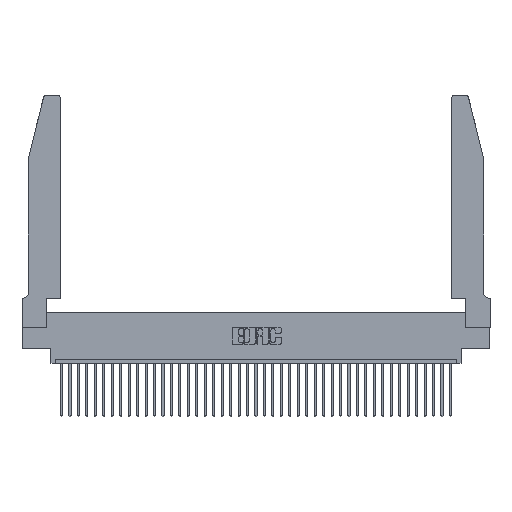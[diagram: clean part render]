
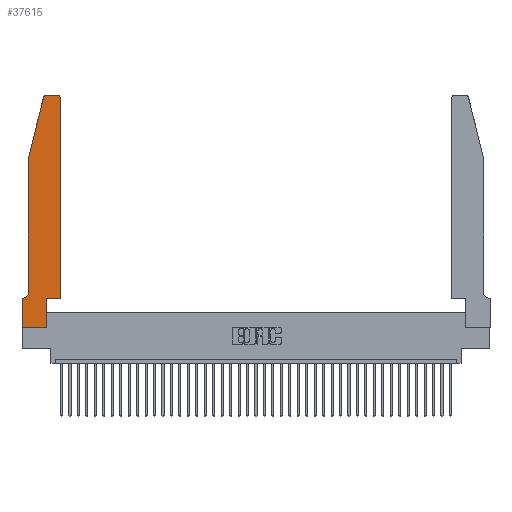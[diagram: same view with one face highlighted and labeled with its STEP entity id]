
A CAD part, top view. The second image highlights one B-rep face of the part: STEP entity #37615.
In plain terms, the highlighted planar face has unit normal (0, 0, 1).
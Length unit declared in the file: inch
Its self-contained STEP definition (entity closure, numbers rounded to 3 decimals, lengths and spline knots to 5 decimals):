
#205 = DIRECTION ( 'NONE',  ( -1., 0., 0. ) ) ;
#298 = EDGE_CURVE ( 'NONE', #4939, #35793, #22184, .T. ) ;
#936 = CARTESIAN_POINT ( 'NONE',  ( 0.0755, 2., 0.37 ) ) ;
#2303 = CARTESIAN_POINT ( 'NONE',  ( 0.284, 2.72, 0.37 ) ) ;
#2521 = CARTESIAN_POINT ( 'NONE',  ( 0.284, 2.75, 0.37 ) ) ;
#3722 = CARTESIAN_POINT ( 'NONE',  ( 0.2865, 0.35, 0.37 ) ) ;
#4431 = VERTEX_POINT ( 'NONE', #35294 ) ;
#4633 = CIRCLE ( 'NONE', #36306, 0.07 ) ;
#4719 = EDGE_CURVE ( 'NONE', #36142, #27491, #20050, .T. ) ;
#4939 = VERTEX_POINT ( 'NONE', #25832 ) ;
#5472 = VECTOR ( 'NONE', #21327, 39.37008 ) ;
#5750 = EDGE_CURVE ( 'NONE', #32243, #20585, #34738, .T. ) ;
#6761 = DIRECTION ( 'NONE',  ( 0., 1., 0. ) ) ;
#7366 = DIRECTION ( 'NONE',  ( -1., 0., 0. ) ) ;
#7475 = PLANE ( 'NONE',  #34757 ) ;
#7503 = DIRECTION ( 'NONE',  ( 1., 0., 0. ) ) ;
#7834 = VECTOR ( 'NONE', #29791, 39.37008 ) ;
#8847 = ORIENTED_EDGE ( 'NONE', *, *, #26041, .T. ) ;
#10154 = CARTESIAN_POINT ( 'NONE',  ( 0.4505, 0.35, 0.37 ) ) ;
#11178 = EDGE_CURVE ( 'NONE', #20585, #12374, #34008, .T. ) ;
#11465 = CARTESIAN_POINT ( 'NONE',  ( 0.0755, 0.35, 0.37 ) ) ;
#11670 = CARTESIAN_POINT ( 'NONE',  ( 0.4505, 0.35, 0.37 ) ) ;
#12374 = VERTEX_POINT ( 'NONE', #31722 ) ;
#12647 = DIRECTION ( 'NONE',  ( 0., -1., 0. ) ) ;
#13326 = EDGE_CURVE ( 'NONE', #36892, #4939, #19471, .T. ) ;
#13401 = VERTEX_POINT ( 'NONE', #14590 ) ;
#13885 = CARTESIAN_POINT ( 'NONE',  ( 0.4205, 2.72, 0.37 ) ) ;
#13896 = EDGE_CURVE ( 'NONE', #13401, #4431, #4633, .T. ) ;
#14023 = DIRECTION ( 'NONE',  ( 1., 0., 0. ) ) ;
#14109 = EDGE_LOOP ( 'NONE', ( #20429, #28844, #33968, #28746, #20818, #35932, #25074, #21228, #8847, #20379, #29897, #29073 ) ) ;
#14533 = LINE ( 'NONE', #11670, #37024 ) ;
#14590 = CARTESIAN_POINT ( 'NONE',  ( 0.0755, 0.42, 0.37 ) ) ;
#15740 = VERTEX_POINT ( 'NONE', #34594 ) ;
#18866 = LINE ( 'NONE', #32473, #7834 ) ;
#19202 = VECTOR ( 'NONE', #205, 39.37008 ) ;
#19305 = DIRECTION ( 'NONE',  ( 0., 0., -1. ) ) ;
#19471 = LINE ( 'NONE', #39380, #24292 ) ;
#20050 = LINE ( 'NONE', #10154, #22392 ) ;
#20379 = ORIENTED_EDGE ( 'NONE', *, *, #4719, .T. ) ;
#20429 = ORIENTED_EDGE ( 'NONE', *, *, #5750, .T. ) ;
#20585 = VERTEX_POINT ( 'NONE', #2521 ) ;
#20818 = ORIENTED_EDGE ( 'NONE', *, *, #13896, .T. ) ;
#21228 = ORIENTED_EDGE ( 'NONE', *, *, #298, .T. ) ;
#21327 = DIRECTION ( 'NONE',  ( 1., 0., 0. ) ) ;
#21542 = CARTESIAN_POINT ( 'NONE',  ( 0.2865, 0.35, 0.37 ) ) ;
#21628 = CARTESIAN_POINT ( 'NONE',  ( 0.4505, 0.35, 0.37 ) ) ;
#21789 = VECTOR ( 'NONE', #6761, 39.37008 ) ;
#22184 = LINE ( 'NONE', #36302, #5472 ) ;
#22392 = VECTOR ( 'NONE', #7503, 39.37008 ) ;
#22797 = VERTEX_POINT ( 'NONE', #24919 ) ;
#23304 = VECTOR ( 'NONE', #7366, 39.37008 ) ;
#23451 = DIRECTION ( 'NONE',  ( 0., 0., 1. ) ) ;
#23716 = DIRECTION ( 'NONE',  ( 0., 0., 1. ) ) ;
#23844 = AXIS2_PLACEMENT_3D ( 'NONE', #2303, #23716, #39201 ) ;
#24028 = DIRECTION ( 'NONE',  ( 0., -1., 0. ) ) ;
#24292 = VECTOR ( 'NONE', #24028, 39.37008 ) ;
#24919 = CARTESIAN_POINT ( 'NONE',  ( 0.0755, 2., 0.37 ) ) ;
#25063 = CARTESIAN_POINT ( 'NONE',  ( 0.0055, 0.42, 0.37 ) ) ;
#25074 = ORIENTED_EDGE ( 'NONE', *, *, #13326, .T. ) ;
#25832 = CARTESIAN_POINT ( 'NONE',  ( 0., 0., 0.37 ) ) ;
#25899 = CARTESIAN_POINT ( 'NONE',  ( 0.2605, 2.75, 0.37 ) ) ;
#26041 = EDGE_CURVE ( 'NONE', #35793, #36142, #29985, .T. ) ;
#26380 = EDGE_CURVE ( 'NONE', #22797, #13401, #39008, .T. ) ;
#26626 = VECTOR ( 'NONE', #12647, 39.37008 ) ;
#27491 = VERTEX_POINT ( 'NONE', #21628 ) ;
#27518 = DIRECTION ( 'NONE',  ( 0., 1., 0. ) ) ;
#28248 = FACE_OUTER_BOUND ( 'NONE', #14109, .T. ) ;
#28746 = ORIENTED_EDGE ( 'NONE', *, *, #26380, .T. ) ;
#28818 = CARTESIAN_POINT ( 'NONE',  ( 0., 0.35, 0.37 ) ) ;
#28844 = ORIENTED_EDGE ( 'NONE', *, *, #11178, .T. ) ;
#29073 = ORIENTED_EDGE ( 'NONE', *, *, #38375, .T. ) ;
#29791 = DIRECTION ( 'NONE',  ( -0.239, -0.971, 0. ) ) ;
#29897 = ORIENTED_EDGE ( 'NONE', *, *, #35470, .T. ) ;
#29985 = LINE ( 'NONE', #3722, #21789 ) ;
#30277 = LINE ( 'NONE', #11465, #19202 ) ;
#31722 = CARTESIAN_POINT ( 'NONE',  ( 0.25487, 2.72718, 0.37 ) ) ;
#32243 = VERTEX_POINT ( 'NONE', #38603 ) ;
#32473 = CARTESIAN_POINT ( 'NONE',  ( 0.0755, 2., 0.37 ) ) ;
#33533 = CIRCLE ( 'NONE', #33772, 0.03 ) ;
#33772 = AXIS2_PLACEMENT_3D ( 'NONE', #13885, #23451, #14023 ) ;
#33968 = ORIENTED_EDGE ( 'NONE', *, *, #39501, .T. ) ;
#34008 = CIRCLE ( 'NONE', #23844, 0.03 ) ;
#34594 = CARTESIAN_POINT ( 'NONE',  ( 0.4505, 2.72, 0.37 ) ) ;
#34713 = CARTESIAN_POINT ( 'NONE',  ( 0., 0.35, 0.37 ) ) ;
#34738 = LINE ( 'NONE', #25899, #23304 ) ;
#34757 = AXIS2_PLACEMENT_3D ( 'NONE', #28818, #38139, #35206 ) ;
#34938 = CARTESIAN_POINT ( 'NONE',  ( 0.2865, 0., 0.37 ) ) ;
#35206 = DIRECTION ( 'NONE',  ( 1., 0., 0. ) ) ;
#35294 = CARTESIAN_POINT ( 'NONE',  ( 0.0055, 0.35, 0.37 ) ) ;
#35470 = EDGE_CURVE ( 'NONE', #27491, #15740, #14533, .T. ) ;
#35793 = VERTEX_POINT ( 'NONE', #34938 ) ;
#35932 = ORIENTED_EDGE ( 'NONE', *, *, #36543, .T. ) ;
#36142 = VERTEX_POINT ( 'NONE', #21542 ) ;
#36302 = CARTESIAN_POINT ( 'NONE',  ( 0., 0., 0.37 ) ) ;
#36306 = AXIS2_PLACEMENT_3D ( 'NONE', #25063, #19305, #37204 ) ;
#36543 = EDGE_CURVE ( 'NONE', #4431, #36892, #30277, .T. ) ;
#36892 = VERTEX_POINT ( 'NONE', #34713 ) ;
#37024 = VECTOR ( 'NONE', #27518, 39.37008 ) ;
#37204 = DIRECTION ( 'NONE',  ( -1., 0., 0. ) ) ;
#37615 = ADVANCED_FACE ( 'NONE', ( #28248 ), #7475, .T. ) ;
#38139 = DIRECTION ( 'NONE',  ( 0., 0., 1. ) ) ;
#38375 = EDGE_CURVE ( 'NONE', #15740, #32243, #33533, .T. ) ;
#38603 = CARTESIAN_POINT ( 'NONE',  ( 0.4205, 2.75, 0.37 ) ) ;
#39008 = LINE ( 'NONE', #936, #26626 ) ;
#39201 = DIRECTION ( 'NONE',  ( 1., 0., 0. ) ) ;
#39380 = CARTESIAN_POINT ( 'NONE',  ( 0., 0., 0.37 ) ) ;
#39501 = EDGE_CURVE ( 'NONE', #12374, #22797, #18866, .T. ) ;
